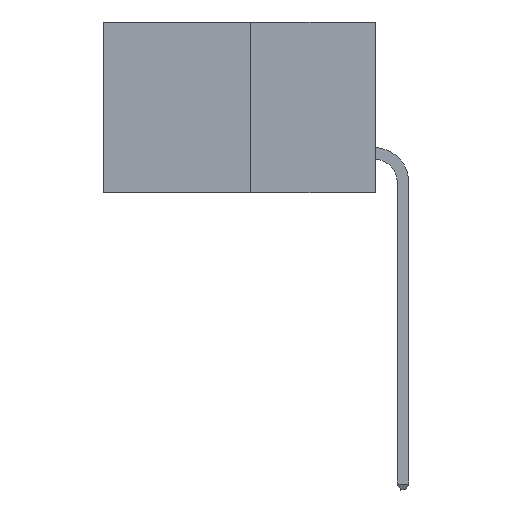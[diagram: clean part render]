
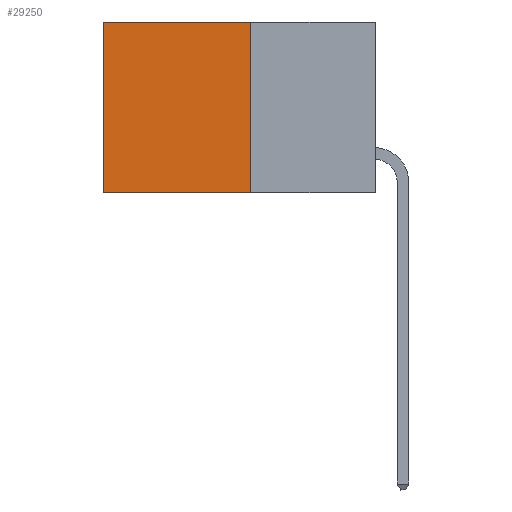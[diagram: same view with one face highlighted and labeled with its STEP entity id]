
A CAD part, left-side view. The second image highlights one B-rep face of the part: STEP entity #29250.
In plain terms, the highlighted planar face has unit normal (-1, 0, 0).
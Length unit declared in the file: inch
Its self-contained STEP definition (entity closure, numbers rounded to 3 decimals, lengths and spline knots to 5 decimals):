
#1259 = DIRECTION ( 'NONE',  ( 0., 1., 0. ) ) ;
#1600 = VECTOR ( 'NONE', #24511, 39.37008 ) ;
#2411 = LINE ( 'NONE', #14626, #1600 ) ;
#3079 = EDGE_CURVE ( 'NONE', #7637, #30622, #8457, .T. ) ;
#3702 = VECTOR ( 'NONE', #1259, 39.37008 ) ;
#3707 = VECTOR ( 'NONE', #9121, 39.37008 ) ;
#4764 = EDGE_CURVE ( 'NONE', #10133, #14790, #2411, .T. ) ;
#5445 = CARTESIAN_POINT ( 'NONE',  ( 0.277, 0.27, -0.37 ) ) ;
#6518 = EDGE_CURVE ( 'NONE', #7637, #10133, #9595, .T. ) ;
#7637 = VERTEX_POINT ( 'NONE', #10042 ) ;
#8457 = LINE ( 'NONE', #17881, #20113 ) ;
#9121 = DIRECTION ( 'NONE',  ( 0., 1., 0. ) ) ;
#9595 = LINE ( 'NONE', #31879, #3707 ) ;
#10042 = CARTESIAN_POINT ( 'NONE',  ( 0.277, 0.27, 0. ) ) ;
#10133 = VERTEX_POINT ( 'NONE', #25487 ) ;
#11848 = ORIENTED_EDGE ( 'NONE', *, *, #26787, .F. ) ;
#12481 = PLANE ( 'NONE',  #26188 ) ;
#12926 = DIRECTION ( 'NONE',  ( 0., 0., -1. ) ) ;
#12939 = EDGE_LOOP ( 'NONE', ( #31607, #11848, #19013, #22741 ) ) ;
#13885 = CARTESIAN_POINT ( 'NONE',  ( 0.277, 0.27, -0.37 ) ) ;
#14626 = CARTESIAN_POINT ( 'NONE',  ( 0.277, 0.59, -0.37 ) ) ;
#14790 = VERTEX_POINT ( 'NONE', #31364 ) ;
#14958 = DIRECTION ( 'NONE',  ( 0., 0., -1. ) ) ;
#17593 = FACE_OUTER_BOUND ( 'NONE', #12939, .T. ) ;
#17787 = LINE ( 'NONE', #13885, #3702 ) ;
#17881 = CARTESIAN_POINT ( 'NONE',  ( 0.277, 0.27, -0.37 ) ) ;
#19013 = ORIENTED_EDGE ( 'NONE', *, *, #3079, .F. ) ;
#20113 = VECTOR ( 'NONE', #12926, 39.37008 ) ;
#22741 = ORIENTED_EDGE ( 'NONE', *, *, #6518, .T. ) ;
#24511 = DIRECTION ( 'NONE',  ( 0., 0., -1. ) ) ;
#25487 = CARTESIAN_POINT ( 'NONE',  ( 0.277, 0.59, 0. ) ) ;
#26188 = AXIS2_PLACEMENT_3D ( 'NONE', #27265, #29763, #14958 ) ;
#26787 = EDGE_CURVE ( 'NONE', #30622, #14790, #17787, .T. ) ;
#27265 = CARTESIAN_POINT ( 'NONE',  ( 0.277, 0.27, -0.37 ) ) ;
#29250 = ADVANCED_FACE ( 'NONE', ( #17593 ), #12481, .F. ) ;
#29763 = DIRECTION ( 'NONE',  ( 1., 0., 0. ) ) ;
#30622 = VERTEX_POINT ( 'NONE', #5445 ) ;
#31364 = CARTESIAN_POINT ( 'NONE',  ( 0.277, 0.59, -0.37 ) ) ;
#31607 = ORIENTED_EDGE ( 'NONE', *, *, #4764, .T. ) ;
#31879 = CARTESIAN_POINT ( 'NONE',  ( 0.277, 0.27, 0. ) ) ;
